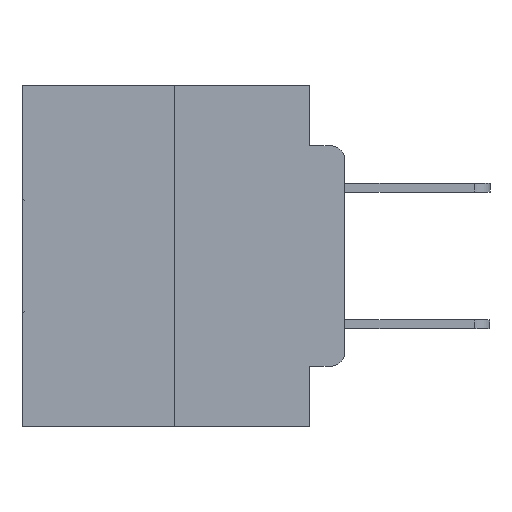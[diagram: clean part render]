
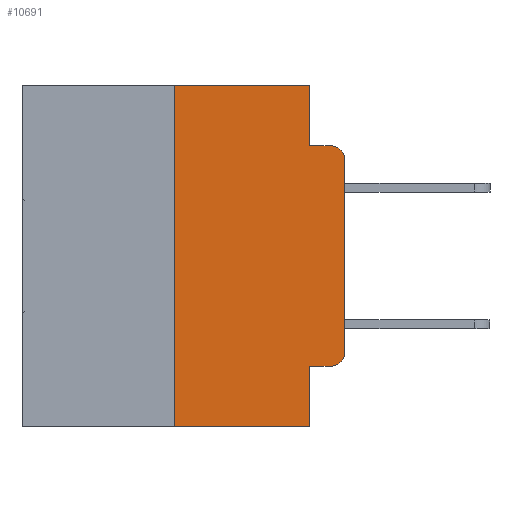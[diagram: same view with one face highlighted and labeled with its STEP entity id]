
A CAD part, left-side view. The second image highlights one B-rep face of the part: STEP entity #10691.
In plain terms, the highlighted planar face has unit normal (-1, 0, 0).
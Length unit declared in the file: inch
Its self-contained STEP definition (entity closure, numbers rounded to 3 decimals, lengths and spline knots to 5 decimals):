
#270 = EDGE_CURVE ( 'NONE', #4254, #9782, #1514, .T. ) ;
#792 = CARTESIAN_POINT ( 'NONE',  ( 0., 0.051, 0. ) ) ;
#1514 = LINE ( 'NONE', #19210, #6162 ) ;
#1526 = VECTOR ( 'NONE', #8411, 39.37008 ) ;
#1831 = DIRECTION ( 'NONE',  ( 0., -1., 0. ) ) ;
#2598 = CARTESIAN_POINT ( 'NONE',  ( 0., 0.473, 0. ) ) ;
#2614 = CIRCLE ( 'NONE', #10453, 0.02 ) ;
#3185 = VERTEX_POINT ( 'NONE', #13947 ) ;
#3411 = VERTEX_POINT ( 'NONE', #6931 ) ;
#3416 = EDGE_CURVE ( 'NONE', #18473, #3185, #23857, .T. ) ;
#3509 = FACE_OUTER_BOUND ( 'NONE', #7003, .T. ) ;
#3732 = VERTEX_POINT ( 'NONE', #16250 ) ;
#4254 = VERTEX_POINT ( 'NONE', #12574 ) ;
#4456 = VECTOR ( 'NONE', #24481, 39.37008 ) ;
#4489 = EDGE_CURVE ( 'NONE', #3732, #21680, #14633, .T. ) ;
#4745 = EDGE_CURVE ( 'NONE', #18473, #9782, #12843, .T. ) ;
#5945 = EDGE_CURVE ( 'NONE', #21307, #12909, #27629, .T. ) ;
#6162 = VECTOR ( 'NONE', #19360, 39.37008 ) ;
#6496 = ORIENTED_EDGE ( 'NONE', *, *, #24581, .F. ) ;
#6654 = CARTESIAN_POINT ( 'NONE',  ( 0., 0.25, 0. ) ) ;
#6899 = DIRECTION ( 'NONE',  ( 0., 0., 1. ) ) ;
#6931 = CARTESIAN_POINT ( 'NONE',  ( 0., 0.02, -0.4115 ) ) ;
#7003 = EDGE_LOOP ( 'NONE', ( #21339, #15913, #14517, #7195, #6496, #10992, #10291, #20682, #19338, #27861 ) ) ;
#7195 = ORIENTED_EDGE ( 'NONE', *, *, #28201, .F. ) ;
#7442 = EDGE_CURVE ( 'NONE', #21680, #12909, #2614, .T. ) ;
#7573 = LINE ( 'NONE', #12804, #1526 ) ;
#7626 = LINE ( 'NONE', #792, #12838 ) ;
#7674 = VERTEX_POINT ( 'NONE', #9140 ) ;
#7733 = CARTESIAN_POINT ( 'NONE',  ( 0., 0.02, -0.0885 ) ) ;
#7974 = VECTOR ( 'NONE', #1831, 39.37008 ) ;
#8381 = CARTESIAN_POINT ( 'NONE',  ( 0., 0.02, -0.1085 ) ) ;
#8411 = DIRECTION ( 'NONE',  ( 0., -1., 0. ) ) ;
#8532 = CARTESIAN_POINT ( 'NONE',  ( 0., 0.051, -0.4115 ) ) ;
#9140 = CARTESIAN_POINT ( 'NONE',  ( 0., 0.051, 0. ) ) ;
#9424 = PLANE ( 'NONE',  #23941 ) ;
#9782 = VERTEX_POINT ( 'NONE', #12595 ) ;
#10291 = ORIENTED_EDGE ( 'NONE', *, *, #4745, .T. ) ;
#10453 = AXIS2_PLACEMENT_3D ( 'NONE', #8381, #23743, #10620 ) ;
#10620 = DIRECTION ( 'NONE',  ( 0., 0., -1. ) ) ;
#10691 = ADVANCED_FACE ( 'NONE', ( #3509 ), #9424, .F. ) ;
#10707 = CARTESIAN_POINT ( 'NONE',  ( 0., 0., 0. ) ) ;
#10992 = ORIENTED_EDGE ( 'NONE', *, *, #3416, .F. ) ;
#11685 = DIRECTION ( 'NONE',  ( 0., 0., -1. ) ) ;
#12574 = CARTESIAN_POINT ( 'NONE',  ( 0., 0.051, -0.4115 ) ) ;
#12595 = CARTESIAN_POINT ( 'NONE',  ( 0., 0.051, -0.5 ) ) ;
#12782 = CARTESIAN_POINT ( 'NONE',  ( 0., 0.02, -0.3915 ) ) ;
#12804 = CARTESIAN_POINT ( 'NONE',  ( 0., 0.473, 0. ) ) ;
#12829 = CARTESIAN_POINT ( 'NONE',  ( 0., 0.051, -0.0885 ) ) ;
#12838 = VECTOR ( 'NONE', #18862, 39.37008 ) ;
#12843 = LINE ( 'NONE', #19138, #18093 ) ;
#12909 = VERTEX_POINT ( 'NONE', #7733 ) ;
#12934 = CARTESIAN_POINT ( 'NONE',  ( 0., 0.25, -0.5 ) ) ;
#13942 = LINE ( 'NONE', #8532, #7974 ) ;
#13947 = CARTESIAN_POINT ( 'NONE',  ( 0., 0.25, 0. ) ) ;
#14517 = ORIENTED_EDGE ( 'NONE', *, *, #5945, .F. ) ;
#14633 = LINE ( 'NONE', #10707, #25443 ) ;
#15038 = DIRECTION ( 'NONE',  ( 0., 0., -1. ) ) ;
#15913 = ORIENTED_EDGE ( 'NONE', *, *, #7442, .T. ) ;
#16250 = CARTESIAN_POINT ( 'NONE',  ( 0., 0., -0.3915 ) ) ;
#16374 = CARTESIAN_POINT ( 'NONE',  ( 0., 0.051, -0.0885 ) ) ;
#16643 = DIRECTION ( 'NONE',  ( 0., -1., 0. ) ) ;
#18093 = VECTOR ( 'NONE', #16643, 39.37008 ) ;
#18473 = VERTEX_POINT ( 'NONE', #12934 ) ;
#18854 = VECTOR ( 'NONE', #6899, 39.37008 ) ;
#18862 = DIRECTION ( 'NONE',  ( 0., 0., -1. ) ) ;
#19138 = CARTESIAN_POINT ( 'NONE',  ( 0., 0.473, -0.5 ) ) ;
#19210 = CARTESIAN_POINT ( 'NONE',  ( 0., 0.051, 0. ) ) ;
#19338 = ORIENTED_EDGE ( 'NONE', *, *, #19821, .T. ) ;
#19360 = DIRECTION ( 'NONE',  ( 0., 0., -1. ) ) ;
#19821 = EDGE_CURVE ( 'NONE', #4254, #3411, #13942, .T. ) ;
#20682 = ORIENTED_EDGE ( 'NONE', *, *, #270, .F. ) ;
#21307 = VERTEX_POINT ( 'NONE', #16374 ) ;
#21339 = ORIENTED_EDGE ( 'NONE', *, *, #4489, .T. ) ;
#21680 = VERTEX_POINT ( 'NONE', #22510 ) ;
#21841 = DIRECTION ( 'NONE',  ( 0., 0., 1. ) ) ;
#22510 = CARTESIAN_POINT ( 'NONE',  ( 0., 0., -0.1085 ) ) ;
#22615 = EDGE_CURVE ( 'NONE', #3411, #3732, #26837, .T. ) ;
#23743 = DIRECTION ( 'NONE',  ( -1., 0., 0. ) ) ;
#23857 = LINE ( 'NONE', #6654, #18854 ) ;
#23941 = AXIS2_PLACEMENT_3D ( 'NONE', #2598, #24738, #11685 ) ;
#24481 = DIRECTION ( 'NONE',  ( 0., -1., 0. ) ) ;
#24581 = EDGE_CURVE ( 'NONE', #3185, #7674, #7573, .T. ) ;
#24738 = DIRECTION ( 'NONE',  ( 1., 0., 0. ) ) ;
#25443 = VECTOR ( 'NONE', #21841, 39.37008 ) ;
#25857 = AXIS2_PLACEMENT_3D ( 'NONE', #12782, #27857, #15038 ) ;
#26837 = CIRCLE ( 'NONE', #25857, 0.02 ) ;
#27629 = LINE ( 'NONE', #12829, #4456 ) ;
#27857 = DIRECTION ( 'NONE',  ( -1., 0., 0. ) ) ;
#27861 = ORIENTED_EDGE ( 'NONE', *, *, #22615, .T. ) ;
#28201 = EDGE_CURVE ( 'NONE', #7674, #21307, #7626, .T. ) ;
